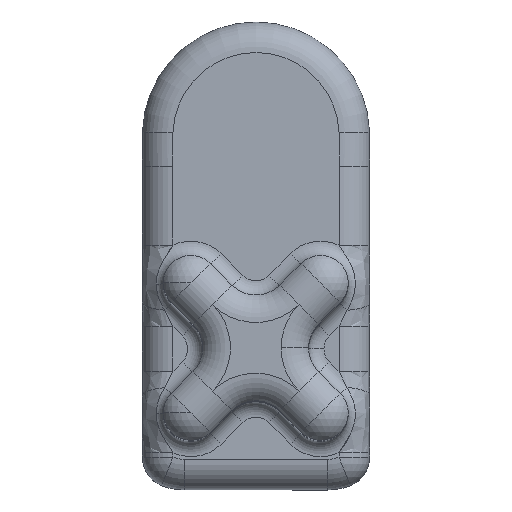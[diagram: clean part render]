
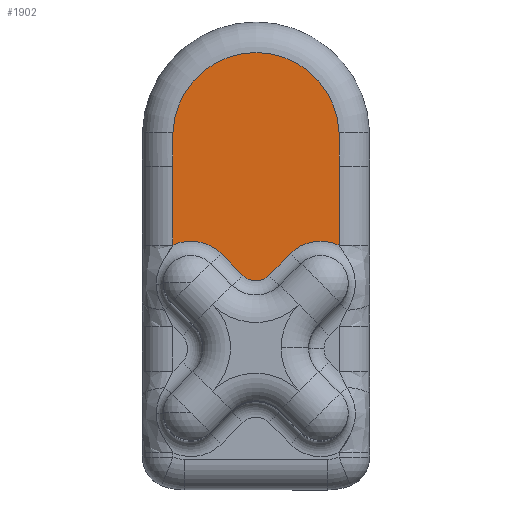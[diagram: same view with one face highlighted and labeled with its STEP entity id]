
A CAD part, top view. The second image highlights one B-rep face of the part: STEP entity #1902.
In plain terms, the highlighted planar face has unit normal (0, 0, 1).
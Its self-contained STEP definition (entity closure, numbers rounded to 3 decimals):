
#128 = CIRCLE ( 'NONE', #3843, 7. ) ;
#246 = DIRECTION ( 'NONE',  ( 0., 1., 0. ) ) ;
#292 = CIRCLE ( 'NONE', #1489, 3. ) ;
#299 = EDGE_CURVE ( 'NONE', #4609, #3515, #3593, .T. ) ;
#324 = ORIENTED_EDGE ( 'NONE', *, *, #4726, .T. ) ;
#346 = LINE ( 'NONE', #4911, #5346 ) ;
#600 = VERTEX_POINT ( 'NONE', #3490 ) ;
#608 = ORIENTED_EDGE ( 'NONE', *, *, #4930, .T. ) ;
#627 = VERTEX_POINT ( 'NONE', #4447 ) ;
#630 = AXIS2_PLACEMENT_3D ( 'NONE', #4649, #1756, #5144 ) ;
#737 = EDGE_CURVE ( 'NONE', #627, #4609, #4481, .T. ) ;
#767 = VERTEX_POINT ( 'NONE', #4558 ) ;
#819 = AXIS2_PLACEMENT_3D ( 'NONE', #4734, #1828, #5215 ) ;
#913 = CARTESIAN_POINT ( 'NONE',  ( -32.829, 15.112, -22.818 ) ) ;
#934 = CARTESIAN_POINT ( 'NONE',  ( -20.101, 16.527, -22.818 ) ) ;
#973 = VERTEX_POINT ( 'NONE', #934 ) ;
#1027 = LINE ( 'NONE', #5479, #4741 ) ;
#1080 = LINE ( 'NONE', #4691, #4793 ) ;
#1113 = DIRECTION ( 'NONE',  ( 0.707, -0.707, 0. ) ) ;
#1175 = CARTESIAN_POINT ( 'NONE',  ( -8.618, 39.361, -22.818 ) ) ;
#1189 = EDGE_CURVE ( 'NONE', #4667, #627, #4256, .T. ) ;
#1380 = EDGE_CURVE ( 'NONE', #973, #5691, #1080, .T. ) ;
#1409 = DIRECTION ( 'NONE',  ( -1., 0., 0. ) ) ;
#1489 = AXIS2_PLACEMENT_3D ( 'NONE', #1856, #5247, #2338 ) ;
#1495 = LINE ( 'NONE', #2151, #5203 ) ;
#1607 = AXIS2_PLACEMENT_3D ( 'NONE', #1649, #5032, #2125 ) ;
#1649 = CARTESIAN_POINT ( 'NONE',  ( -11.616, 15.112, -22.818 ) ) ;
#1756 = DIRECTION ( 'NONE',  ( 0., 0., -1. ) ) ;
#1828 = DIRECTION ( 'NONE',  ( 0., 0., 1. ) ) ;
#1856 = CARTESIAN_POINT ( 'NONE',  ( -22.222, 18.648, -22.818 ) ) ;
#1902 = ADVANCED_FACE ( 'NONE', ( #1983 ), #5577, .F. ) ;
#1956 = EDGE_CURVE ( 'NONE', #5691, #4667, #4246, .T. ) ;
#1983 = FACE_OUTER_BOUND ( 'NONE', #5742, .T. ) ;
#2010 = DIRECTION ( 'NONE',  ( 0., -1., 0. ) ) ;
#2125 = DIRECTION ( 'NONE',  ( -1., 0., 0. ) ) ;
#2139 = EDGE_CURVE ( 'NONE', #5729, #973, #292, .T. ) ;
#2151 = CARTESIAN_POINT ( 'NONE',  ( -35.751, 39.361, -22.818 ) ) ;
#2338 = DIRECTION ( 'NONE',  ( -1., 0., 0. ) ) ;
#2545 = CARTESIAN_POINT ( 'NONE',  ( -8.618, 39.838, -22.818 ) ) ;
#2704 = CARTESIAN_POINT ( 'NONE',  ( -8.618, 39.361, -22.818 ) ) ;
#2938 = EDGE_CURVE ( 'NONE', #600, #767, #128, .T. ) ;
#2960 = ORIENTED_EDGE ( 'NONE', *, *, #1956, .T. ) ;
#2981 = VECTOR ( 'NONE', #5590, 1000. ) ;
#3133 = CARTESIAN_POINT ( 'NONE',  ( -24.344, 16.527, -22.818 ) ) ;
#3490 = CARTESIAN_POINT ( 'NONE',  ( -35.751, 21.473, -22.818 ) ) ;
#3515 = VERTEX_POINT ( 'NONE', #4335 ) ;
#3593 = CIRCLE ( 'NONE', #819, 13.575 ) ;
#3621 = DIRECTION ( 'NONE',  ( 0., -1., 0. ) ) ;
#3843 = AXIS2_PLACEMENT_3D ( 'NONE', #913, #4293, #1409 ) ;
#3868 = CARTESIAN_POINT ( 'NONE',  ( -35.751, 34.373, -22.818 ) ) ;
#4059 = CARTESIAN_POINT ( 'NONE',  ( -8.618, 21.438, -22.818 ) ) ;
#4203 = DIRECTION ( 'NONE',  ( 0.707, 0.707, 0. ) ) ;
#4246 = CIRCLE ( 'NONE', #1607, 7. ) ;
#4256 = LINE ( 'NONE', #2704, #2981 ) ;
#4293 = DIRECTION ( 'NONE',  ( 0., 0., -1. ) ) ;
#4323 = ORIENTED_EDGE ( 'NONE', *, *, #737, .T. ) ;
#4335 = CARTESIAN_POINT ( 'NONE',  ( -35.751, 39.838, -22.818 ) ) ;
#4447 = CARTESIAN_POINT ( 'NONE',  ( -8.618, 34.373, -22.818 ) ) ;
#4481 = LINE ( 'NONE', #1175, #4797 ) ;
#4558 = CARTESIAN_POINT ( 'NONE',  ( -27.879, 20.062, -22.818 ) ) ;
#4604 = ORIENTED_EDGE ( 'NONE', *, *, #5490, .T. ) ;
#4609 = VERTEX_POINT ( 'NONE', #2545 ) ;
#4649 = CARTESIAN_POINT ( 'NONE',  ( -22.184, 39.361, -22.818 ) ) ;
#4667 = VERTEX_POINT ( 'NONE', #4059 ) ;
#4691 = CARTESIAN_POINT ( 'NONE',  ( -16.566, 20.062, -22.818 ) ) ;
#4726 = EDGE_CURVE ( 'NONE', #5902, #600, #1495, .T. ) ;
#4734 = CARTESIAN_POINT ( 'NONE',  ( -22.184, 39.361, -22.818 ) ) ;
#4741 = VECTOR ( 'NONE', #1113, 1000. ) ;
#4793 = VECTOR ( 'NONE', #4203, 1000. ) ;
#4797 = VECTOR ( 'NONE', #246, 1000. ) ;
#4911 = CARTESIAN_POINT ( 'NONE',  ( -35.751, 39.361, -22.818 ) ) ;
#4930 = EDGE_CURVE ( 'NONE', #767, #5729, #1027, .T. ) ;
#5028 = ORIENTED_EDGE ( 'NONE', *, *, #1189, .T. ) ;
#5032 = DIRECTION ( 'NONE',  ( 0., 0., -1. ) ) ;
#5144 = DIRECTION ( 'NONE',  ( 0., -1., 0. ) ) ;
#5203 = VECTOR ( 'NONE', #3621, 1000. ) ;
#5215 = DIRECTION ( 'NONE',  ( -1., 0., 0. ) ) ;
#5236 = ORIENTED_EDGE ( 'NONE', *, *, #2938, .T. ) ;
#5241 = ORIENTED_EDGE ( 'NONE', *, *, #2139, .T. ) ;
#5247 = DIRECTION ( 'NONE',  ( 0., 0., 1. ) ) ;
#5346 = VECTOR ( 'NONE', #2010, 1000. ) ;
#5392 = ORIENTED_EDGE ( 'NONE', *, *, #299, .T. ) ;
#5479 = CARTESIAN_POINT ( 'NONE',  ( -24.344, 16.527, -22.818 ) ) ;
#5490 = EDGE_CURVE ( 'NONE', #3515, #5902, #346, .T. ) ;
#5516 = CARTESIAN_POINT ( 'NONE',  ( -16.566, 20.062, -22.818 ) ) ;
#5577 = PLANE ( 'NONE',  #630 ) ;
#5590 = DIRECTION ( 'NONE',  ( 0., 1., 0. ) ) ;
#5691 = VERTEX_POINT ( 'NONE', #5516 ) ;
#5729 = VERTEX_POINT ( 'NONE', #3133 ) ;
#5742 = EDGE_LOOP ( 'NONE', ( #2960, #5028, #4323, #5392, #4604, #324, #5236, #608, #5241, #6221 ) ) ;
#5902 = VERTEX_POINT ( 'NONE', #3868 ) ;
#6221 = ORIENTED_EDGE ( 'NONE', *, *, #1380, .T. ) ;
